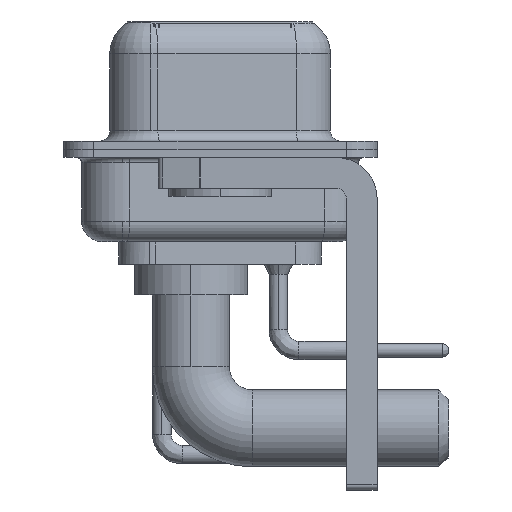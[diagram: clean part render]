
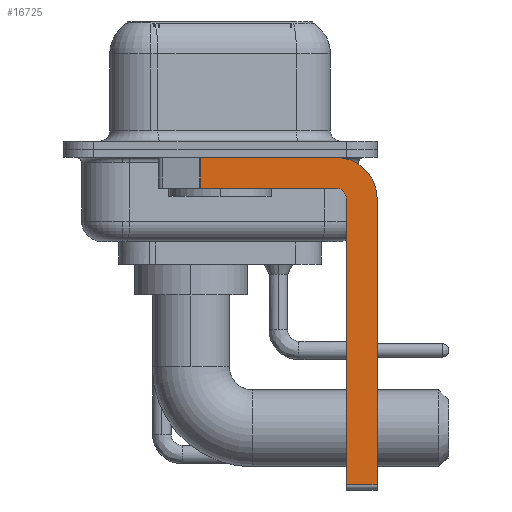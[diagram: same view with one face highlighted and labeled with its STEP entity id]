
A CAD part, left-side view. The second image highlights one B-rep face of the part: STEP entity #16725.
In plain terms, the highlighted planar face has unit normal (-1, 0, 0).
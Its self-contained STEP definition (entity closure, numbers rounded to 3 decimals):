
#1457 = VECTOR ( 'NONE', #28556, 1000. ) ;
#2381 = EDGE_CURVE ( 'NONE', #25281, #19243, #29332, .T. ) ;
#2408 = DIRECTION ( 'NONE',  ( 0., -1., 0. ) ) ;
#2850 = EDGE_CURVE ( 'NONE', #20542, #19243, #9076, .T. ) ;
#3324 = AXIS2_PLACEMENT_3D ( 'NONE', #20196, #7218, #32809 ) ;
#3410 = VECTOR ( 'NONE', #29455, 1000. ) ;
#4357 = FACE_OUTER_BOUND ( 'NONE', #31903, .T. ) ;
#4858 = DIRECTION ( 'NONE',  ( 0., 0., -1. ) ) ;
#4921 = LINE ( 'NONE', #6499, #23966 ) ;
#5429 = ORIENTED_EDGE ( 'NONE', *, *, #2381, .T. ) ;
#5459 = VECTOR ( 'NONE', #2408, 1000. ) ;
#5847 = VERTEX_POINT ( 'NONE', #23286 ) ;
#6499 = CARTESIAN_POINT ( 'NONE',  ( -2.9, 0.978, -1.9 ) ) ;
#6543 = AXIS2_PLACEMENT_3D ( 'NONE', #23995, #17855, #4858 ) ;
#7218 = DIRECTION ( 'NONE',  ( 1., 0., 0. ) ) ;
#7397 = EDGE_CURVE ( 'NONE', #8213, #5847, #4921, .T. ) ;
#8213 = VERTEX_POINT ( 'NONE', #14812 ) ;
#8330 = CIRCLE ( 'NONE', #33043, 0.5 ) ;
#9076 = LINE ( 'NONE', #23909, #3410 ) ;
#9672 = VECTOR ( 'NONE', #21589, 1000. ) ;
#10349 = CARTESIAN_POINT ( 'NONE',  ( -2.9, -7.65, -16.35 ) ) ;
#10522 = CARTESIAN_POINT ( 'NONE',  ( -2.9, -5.65, -1.9 ) ) ;
#10683 = VERTEX_POINT ( 'NONE', #19042 ) ;
#11192 = ORIENTED_EDGE ( 'NONE', *, *, #2850, .F. ) ;
#11976 = DIRECTION ( 'NONE',  ( 0., 0., 1. ) ) ;
#14013 = CARTESIAN_POINT ( 'NONE',  ( -2.9, -5.65, -16.35 ) ) ;
#14812 = CARTESIAN_POINT ( 'NONE',  ( -2.9, 0.978, -0.4 ) ) ;
#15153 = VECTOR ( 'NONE', #28874, 1000. ) ;
#15468 = CARTESIAN_POINT ( 'NONE',  ( -2.9, -6.15, -2.4 ) ) ;
#16725 = ADVANCED_FACE ( 'NONE', ( #4357 ), #22061, .F. ) ;
#16819 = ORIENTED_EDGE ( 'NONE', *, *, #25555, .F. ) ;
#17030 = DIRECTION ( 'NONE',  ( -1., 0., 0. ) ) ;
#17787 = EDGE_CURVE ( 'NONE', #8213, #10683, #33221, .T. ) ;
#17855 = DIRECTION ( 'NONE',  ( 1., 0., 0. ) ) ;
#18348 = CARTESIAN_POINT ( 'NONE',  ( -2.9, -6.15, -16.35 ) ) ;
#18624 = CARTESIAN_POINT ( 'NONE',  ( -2.9, -6.15, -16.6 ) ) ;
#18765 = ORIENTED_EDGE ( 'NONE', *, *, #27348, .F. ) ;
#19042 = CARTESIAN_POINT ( 'NONE',  ( -2.9, -5.65, -0.4 ) ) ;
#19243 = VERTEX_POINT ( 'NONE', #10349 ) ;
#20064 = EDGE_CURVE ( 'NONE', #30002, #23016, #8330, .T. ) ;
#20196 = CARTESIAN_POINT ( 'NONE',  ( -2.9, -5.65, -2.4 ) ) ;
#20542 = VERTEX_POINT ( 'NONE', #22496 ) ;
#21083 = CIRCLE ( 'NONE', #6543, 2. ) ;
#21589 = DIRECTION ( 'NONE',  ( 0., -1., 0. ) ) ;
#21861 = ORIENTED_EDGE ( 'NONE', *, *, #20064, .F. ) ;
#22061 = PLANE ( 'NONE',  #3324 ) ;
#22496 = CARTESIAN_POINT ( 'NONE',  ( -2.9, -7.65, -2.4 ) ) ;
#23016 = VERTEX_POINT ( 'NONE', #31363 ) ;
#23286 = CARTESIAN_POINT ( 'NONE',  ( -2.9, 0.978, -1.9 ) ) ;
#23909 = CARTESIAN_POINT ( 'NONE',  ( -2.9, -7.65, -2.4 ) ) ;
#23948 = EDGE_CURVE ( 'NONE', #25281, #30002, #25859, .T. ) ;
#23966 = VECTOR ( 'NONE', #32426, 1000. ) ;
#23995 = CARTESIAN_POINT ( 'NONE',  ( -2.9, -5.65, -2.4 ) ) ;
#25281 = VERTEX_POINT ( 'NONE', #18348 ) ;
#25488 = CARTESIAN_POINT ( 'NONE',  ( -2.9, 3., -0.4 ) ) ;
#25555 = EDGE_CURVE ( 'NONE', #23016, #5847, #26004, .T. ) ;
#25859 = LINE ( 'NONE', #18624, #1457 ) ;
#26004 = LINE ( 'NONE', #10522, #15153 ) ;
#27062 = ORIENTED_EDGE ( 'NONE', *, *, #17787, .F. ) ;
#27348 = EDGE_CURVE ( 'NONE', #10683, #20542, #21083, .T. ) ;
#28556 = DIRECTION ( 'NONE',  ( 0., 0., 1. ) ) ;
#28874 = DIRECTION ( 'NONE',  ( 0., 1., 0. ) ) ;
#29067 = ORIENTED_EDGE ( 'NONE', *, *, #23948, .F. ) ;
#29189 = ORIENTED_EDGE ( 'NONE', *, *, #7397, .T. ) ;
#29332 = LINE ( 'NONE', #14013, #9672 ) ;
#29455 = DIRECTION ( 'NONE',  ( 0., 0., -1. ) ) ;
#29805 = CARTESIAN_POINT ( 'NONE',  ( -2.9, -5.65, -2.4 ) ) ;
#30002 = VERTEX_POINT ( 'NONE', #15468 ) ;
#31363 = CARTESIAN_POINT ( 'NONE',  ( -2.9, -5.65, -1.9 ) ) ;
#31903 = EDGE_LOOP ( 'NONE', ( #27062, #29189, #16819, #21861, #29067, #5429, #11192, #18765 ) ) ;
#32426 = DIRECTION ( 'NONE',  ( 0., 0., -1. ) ) ;
#32809 = DIRECTION ( 'NONE',  ( 0., 0., -1. ) ) ;
#33043 = AXIS2_PLACEMENT_3D ( 'NONE', #29805, #17030, #11976 ) ;
#33221 = LINE ( 'NONE', #25488, #5459 ) ;
